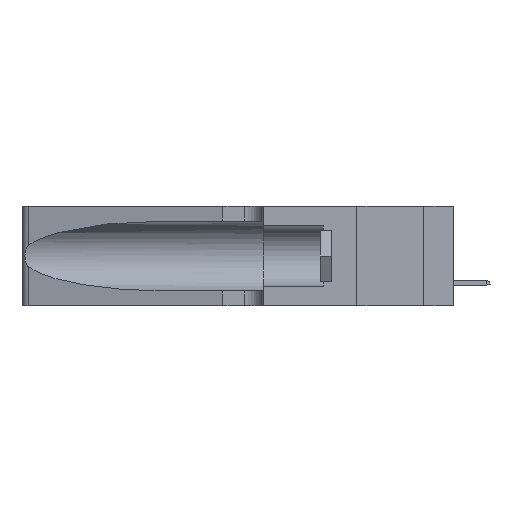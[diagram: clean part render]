
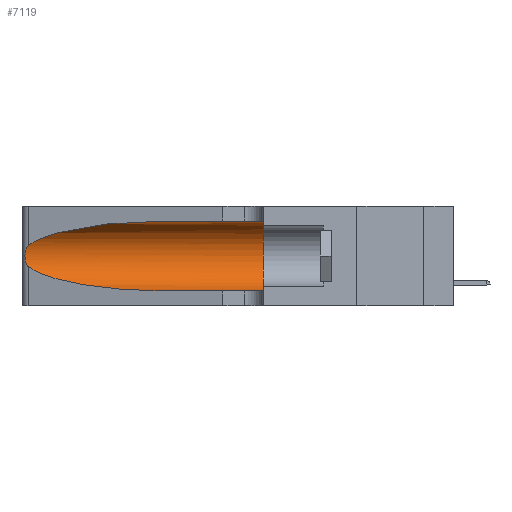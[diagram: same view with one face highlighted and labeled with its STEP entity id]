
A CAD part, left-side view. The second image highlights one B-rep face of the part: STEP entity #7119.
In plain terms, the highlighted cylindrical face has radius 3.308 mm (diameter 6.617 mm), a partial arc.
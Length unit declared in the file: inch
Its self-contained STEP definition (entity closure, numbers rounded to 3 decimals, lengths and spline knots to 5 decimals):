
#475 = VERTEX_POINT ( 'NONE', #4118 ) ;
#1336 = CARTESIAN_POINT ( 'NONE',  ( 0.25487, 1.22718, 0.14631 ) ) ;
#1744 = ORIENTED_EDGE ( 'NONE', *, *, #9308, .T. ) ;
#2046 = CARTESIAN_POINT ( 'NONE',  ( 0.25639, 1.23184, 0.21858 ) ) ;
#2386 = VERTEX_POINT ( 'NONE', #7867 ) ;
#2400 = CARTESIAN_POINT ( 'NONE',  ( 0.25487, 1.22718, 0.22369 ) ) ;
#3295 = CARTESIAN_POINT ( 'NONE',  ( 0.18966, 0.96281, 0.05475 ) ) ;
#3304 = AXIS2_PLACEMENT_3D ( 'NONE', #3911, #11932, #13637 ) ;
#3374 = EDGE_CURVE ( 'NONE', #23494, #2386, #23387, .T. ) ;
#3423 = CARTESIAN_POINT ( 'NONE',  ( 0.1305, 0.72297, 0.05475 ) ) ;
#3857 = CARTESIAN_POINT ( 'NONE',  ( 0.26075, 1.23896, 0.19203 ) ) ;
#3911 = CARTESIAN_POINT ( 'NONE',  ( 0.1305, 1.61858, 0.185 ) ) ;
#4118 = CARTESIAN_POINT ( 'NONE',  ( 0.1305, 0.72297, 0.31525 ) ) ;
#5404 = EDGE_CURVE ( 'NONE', #475, #9076, #7477, .T. ) ;
#5422 = VECTOR ( 'NONE', #25598, 39.37008 ) ;
#5484 = ORIENTED_EDGE ( 'NONE', *, *, #11388, .F. ) ;
#6103 = CARTESIAN_POINT ( 'NONE',  ( 0.25787, 1.23484, 0.2124 ) ) ;
#6232 = CARTESIAN_POINT ( 'NONE',  ( 0.1305, 0.72297, 0.31525 ) ) ;
#6802 =( BOUNDED_CURVE ( )  B_SPLINE_CURVE ( 3, ( #6232, #18762, #20490, #8196 ),
 .UNSPECIFIED., .F., .T. ) 
 B_SPLINE_CURVE_WITH_KNOTS ( ( 4, 4 ),
 ( 1.5708, 2.84003 ),
 .UNSPECIFIED. ) 
 CURVE ( )  GEOMETRIC_REPRESENTATION_ITEM ( )  RATIONAL_B_SPLINE_CURVE ( ( 1., 0.87, 0.87, 1. ) ) 
 REPRESENTATION_ITEM ( '' )  );
#7119 = ADVANCED_FACE ( 'NONE', ( #9567 ), #21875, .F. ) ;
#7477 = LINE ( 'NONE', #17575, #5422 ) ;
#7536 = CARTESIAN_POINT ( 'NONE',  ( 0.25555, 1.22993, 0.14849 ) ) ;
#7867 = CARTESIAN_POINT ( 'NONE',  ( 0.25487, 1.22718, 0.14631 ) ) ;
#7968 = ORIENTED_EDGE ( 'NONE', *, *, #3374, .T. ) ;
#8071 = CARTESIAN_POINT ( 'NONE',  ( 0.26017, 1.23833, 0.17102 ) ) ;
#8110 = AXIS2_PLACEMENT_3D ( 'NONE', #9721, #17441, #15479 ) ;
#8196 = CARTESIAN_POINT ( 'NONE',  ( 0.25487, 1.22718, 0.22369 ) ) ;
#9076 = VERTEX_POINT ( 'NONE', #9379 ) ;
#9308 = EDGE_CURVE ( 'NONE', #475, #23494, #6802, .T. ) ;
#9379 = CARTESIAN_POINT ( 'NONE',  ( 0.1305, 0.35, 0.31525 ) ) ;
#9495 = VERTEX_POINT ( 'NONE', #3423 ) ;
#9567 = FACE_OUTER_BOUND ( 'NONE', #10368, .T. ) ;
#9721 = CARTESIAN_POINT ( 'NONE',  ( 0.1305, 0.35, 0.185 ) ) ;
#9776 = CARTESIAN_POINT ( 'NONE',  ( 0.25854, 1.2359, 0.20912 ) ) ;
#10049 = CARTESIAN_POINT ( 'NONE',  ( 0.26018, 1.23835, 0.19895 ) ) ;
#10368 = EDGE_LOOP ( 'NONE', ( #1744, #7968, #13722, #21059, #5484, #24565 ) ) ;
#10680 = DIRECTION ( 'NONE',  ( 0., -1., 0. ) ) ;
#11315 = CARTESIAN_POINT ( 'NONE',  ( 0.1305, 0.72297, 0.05475 ) ) ;
#11388 = EDGE_CURVE ( 'NONE', #9076, #25718, #11872, .T. ) ;
#11872 = CIRCLE ( 'NONE', #8110, 0.13025 ) ;
#11932 = DIRECTION ( 'NONE',  ( 0., -1., 0. ) ) ;
#12070 = EDGE_CURVE ( 'NONE', #9495, #25718, #12662, .T. ) ;
#12147 = CARTESIAN_POINT ( 'NONE',  ( 0.25789, 1.23486, 0.15765 ) ) ;
#12662 = LINE ( 'NONE', #18537, #15696 ) ;
#13637 = DIRECTION ( 'NONE',  ( 0., 0., -1. ) ) ;
#13722 = ORIENTED_EDGE ( 'NONE', *, *, #20281, .T. ) ;
#14044 =( BOUNDED_CURVE ( )  B_SPLINE_CURVE ( 3, ( #1336, #17858, #3295, #11315 ),
 .UNSPECIFIED., .F., .T. ) 
 B_SPLINE_CURVE_WITH_KNOTS ( ( 4, 4 ),
 ( 3.44316, 4.71239 ),
 .UNSPECIFIED. ) 
 CURVE ( )  GEOMETRIC_REPRESENTATION_ITEM ( )  RATIONAL_B_SPLINE_CURVE ( ( 1., 0.87, 0.87, 1. ) ) 
 REPRESENTATION_ITEM ( '' )  );
#14121 = CARTESIAN_POINT ( 'NONE',  ( 0.25856, 1.23593, 0.16098 ) ) ;
#15479 = DIRECTION ( 'NONE',  ( 0., 0., 1. ) ) ;
#15696 = VECTOR ( 'NONE', #10680, 39.37008 ) ;
#15796 = CARTESIAN_POINT ( 'NONE',  ( 0.26075, 1.23896, 0.178 ) ) ;
#17354 = CARTESIAN_POINT ( 'NONE',  ( 0.1305, 0.35, 0.05475 ) ) ;
#17441 = DIRECTION ( 'NONE',  ( 0., 1., 0. ) ) ;
#17575 = CARTESIAN_POINT ( 'NONE',  ( 0.1305, 1.61858, 0.31525 ) ) ;
#17858 = CARTESIAN_POINT ( 'NONE',  ( 0.2373, 1.15595, 0.08982 ) ) ;
#18537 = CARTESIAN_POINT ( 'NONE',  ( 0.1305, 1.61858, 0.05475 ) ) ;
#18762 = CARTESIAN_POINT ( 'NONE',  ( 0.18966, 0.96281, 0.31525 ) ) ;
#19712 = CARTESIAN_POINT ( 'NONE',  ( 0.25487, 1.22718, 0.22369 ) ) ;
#20115 = CARTESIAN_POINT ( 'NONE',  ( 0.25487, 1.22718, 0.14631 ) ) ;
#20281 = EDGE_CURVE ( 'NONE', #2386, #9495, #14044, .T. ) ;
#20490 = CARTESIAN_POINT ( 'NONE',  ( 0.2373, 1.15595, 0.28018 ) ) ;
#21059 = ORIENTED_EDGE ( 'NONE', *, *, #12070, .T. ) ;
#21817 = CARTESIAN_POINT ( 'NONE',  ( 0.25555, 1.22994, 0.2215 ) ) ;
#21875 = CYLINDRICAL_SURFACE ( 'NONE', #3304, 0.13025 ) ;
#23387 = B_SPLINE_CURVE_WITH_KNOTS ( 'NONE', 3,
 ( #19712, #21817, #2046, #6103, #9776, #10049, #3857, #15796, #8071, #14121, #12147, #23794, #7536, #20115 ),
 .UNSPECIFIED., .F., .F.,
 ( 4, 2, 2, 2, 2, 2, 4 ),
 ( 0., 0.00027, 0.00053, 0.00107, 0.0016, 0.00187, 0.00214 ),
 .UNSPECIFIED. ) ;
#23494 = VERTEX_POINT ( 'NONE', #2400 ) ;
#23794 = CARTESIAN_POINT ( 'NONE',  ( 0.25639, 1.23186, 0.15144 ) ) ;
#24565 = ORIENTED_EDGE ( 'NONE', *, *, #5404, .F. ) ;
#25598 = DIRECTION ( 'NONE',  ( 0., -1., 0. ) ) ;
#25718 = VERTEX_POINT ( 'NONE', #17354 ) ;
